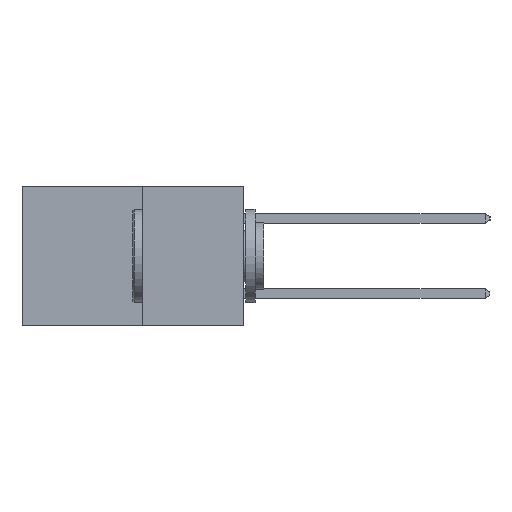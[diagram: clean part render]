
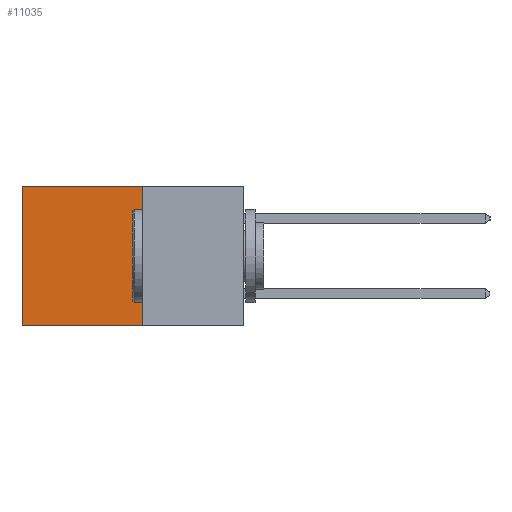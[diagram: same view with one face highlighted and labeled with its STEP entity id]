
A CAD part, left-side view. The second image highlights one B-rep face of the part: STEP entity #11035.
In plain terms, the highlighted planar face has unit normal (-1, 0, 0).
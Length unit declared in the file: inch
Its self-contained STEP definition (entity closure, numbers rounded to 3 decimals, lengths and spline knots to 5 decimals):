
#438 = CARTESIAN_POINT ( 'NONE',  ( 0.277, 0.27, -0.37 ) ) ;
#1131 = EDGE_LOOP ( 'NONE', ( #5815, #4247, #6430, #3436 ) ) ;
#1575 = AXIS2_PLACEMENT_3D ( 'NONE', #438, #13446, #2319 ) ;
#2319 = DIRECTION ( 'NONE',  ( 0., 0., -1. ) ) ;
#3034 = CARTESIAN_POINT ( 'NONE',  ( 0.277, 0.27, 0. ) ) ;
#3436 = ORIENTED_EDGE ( 'NONE', *, *, #10331, .T. ) ;
#3557 = DIRECTION ( 'NONE',  ( 0., 0., -1. ) ) ;
#3674 = CARTESIAN_POINT ( 'NONE',  ( 0.277, 0.27, -0.37 ) ) ;
#4247 = ORIENTED_EDGE ( 'NONE', *, *, #11542, .F. ) ;
#4874 = FACE_OUTER_BOUND ( 'NONE', #1131, .T. ) ;
#5815 = ORIENTED_EDGE ( 'NONE', *, *, #21900, .T. ) ;
#6430 = ORIENTED_EDGE ( 'NONE', *, *, #15920, .F. ) ;
#9265 = VECTOR ( 'NONE', #3557, 39.37008 ) ;
#9377 = DIRECTION ( 'NONE',  ( 0., 0., -1. ) ) ;
#9726 = PLANE ( 'NONE',  #1575 ) ;
#9737 = VERTEX_POINT ( 'NONE', #14841 ) ;
#10331 = EDGE_CURVE ( 'NONE', #18873, #14452, #16208, .T. ) ;
#10802 = DIRECTION ( 'NONE',  ( 0., 1., 0. ) ) ;
#11035 = ADVANCED_FACE ( 'NONE', ( #4874 ), #9726, .F. ) ;
#11106 = VERTEX_POINT ( 'NONE', #13607 ) ;
#11542 = EDGE_CURVE ( 'NONE', #9737, #11106, #18734, .T. ) ;
#11953 = VECTOR ( 'NONE', #9377, 39.37008 ) ;
#12831 = CARTESIAN_POINT ( 'NONE',  ( 0.277, 0.27, -0.37 ) ) ;
#13446 = DIRECTION ( 'NONE',  ( 1., 0., 0. ) ) ;
#13607 = CARTESIAN_POINT ( 'NONE',  ( 0.277, 0.59, -0.37 ) ) ;
#14440 = VECTOR ( 'NONE', #16654, 39.37008 ) ;
#14452 = VERTEX_POINT ( 'NONE', #21931 ) ;
#14841 = CARTESIAN_POINT ( 'NONE',  ( 0.277, 0.27, -0.37 ) ) ;
#15920 = EDGE_CURVE ( 'NONE', #18873, #9737, #18049, .T. ) ;
#16208 = LINE ( 'NONE', #23671, #20512 ) ;
#16653 = CARTESIAN_POINT ( 'NONE',  ( 0.277, 0.59, -0.37 ) ) ;
#16654 = DIRECTION ( 'NONE',  ( 0., 1., 0. ) ) ;
#16870 = LINE ( 'NONE', #16653, #11953 ) ;
#18049 = LINE ( 'NONE', #12831, #9265 ) ;
#18734 = LINE ( 'NONE', #3674, #14440 ) ;
#18873 = VERTEX_POINT ( 'NONE', #3034 ) ;
#20512 = VECTOR ( 'NONE', #10802, 39.37008 ) ;
#21900 = EDGE_CURVE ( 'NONE', #14452, #11106, #16870, .T. ) ;
#21931 = CARTESIAN_POINT ( 'NONE',  ( 0.277, 0.59, 0. ) ) ;
#23671 = CARTESIAN_POINT ( 'NONE',  ( 0.277, 0.27, 0. ) ) ;
